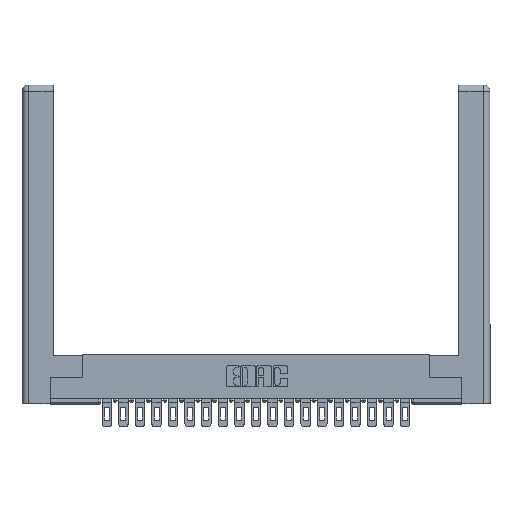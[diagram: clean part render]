
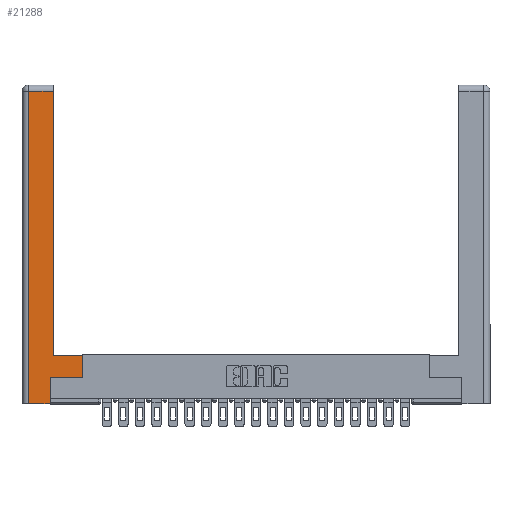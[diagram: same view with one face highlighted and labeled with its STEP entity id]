
A CAD part, top view. The second image highlights one B-rep face of the part: STEP entity #21288.
In plain terms, the highlighted planar face has unit normal (0, 0, 1).
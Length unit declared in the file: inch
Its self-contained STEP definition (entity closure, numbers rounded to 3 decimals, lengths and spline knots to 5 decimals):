
#2 = EDGE_CURVE ( 'NONE', #5353, #17691, #2559, .T. ) ;
#221 = ORIENTED_EDGE ( 'NONE', *, *, #21952, .T. ) ;
#541 = EDGE_CURVE ( 'NONE', #5933, #18225, #8132, .T. ) ;
#936 = VECTOR ( 'NONE', #11601, 39.37008 ) ;
#969 = CARTESIAN_POINT ( 'NONE',  ( 0.0615, 2.94, 0. ) ) ;
#1116 = LINE ( 'NONE', #15059, #15071 ) ;
#1229 = LINE ( 'NONE', #8319, #14444 ) ;
#1489 = CARTESIAN_POINT ( 'NONE',  ( 0.295, 2.94, 0. ) ) ;
#1703 = VECTOR ( 'NONE', #14948, 39.37008 ) ;
#2006 = ORIENTED_EDGE ( 'NONE', *, *, #16409, .T. ) ;
#2559 = LINE ( 'NONE', #12958, #22530 ) ;
#3538 = EDGE_CURVE ( 'NONE', #9638, #11837, #21744, .T. ) ;
#4379 = DIRECTION ( 'NONE',  ( 0., 1., 0. ) ) ;
#4420 = CARTESIAN_POINT ( 'NONE',  ( 0.565, 0.245, 0. ) ) ;
#4484 = CARTESIAN_POINT ( 'NONE',  ( 0.265, 0., 0. ) ) ;
#4649 = CARTESIAN_POINT ( 'NONE',  ( 0.265, 0.245, 0. ) ) ;
#5353 = VERTEX_POINT ( 'NONE', #4420 ) ;
#5506 = CARTESIAN_POINT ( 'NONE',  ( 0.565, 0.45, 0. ) ) ;
#5794 = ORIENTED_EDGE ( 'NONE', *, *, #19524, .T. ) ;
#5933 = VERTEX_POINT ( 'NONE', #22393 ) ;
#6152 = CARTESIAN_POINT ( 'NONE',  ( 0.265, 0., 0. ) ) ;
#7024 = DIRECTION ( 'NONE',  ( 0., 0., -1. ) ) ;
#8132 = LINE ( 'NONE', #4484, #17744 ) ;
#8298 = LINE ( 'NONE', #20510, #1703 ) ;
#8319 = CARTESIAN_POINT ( 'NONE',  ( 0.565, 0.245, 0. ) ) ;
#8575 = VECTOR ( 'NONE', #18726, 39.37008 ) ;
#8745 = PLANE ( 'NONE',  #9283 ) ;
#9079 = CARTESIAN_POINT ( 'NONE',  ( 0., 0., 0. ) ) ;
#9283 = AXIS2_PLACEMENT_3D ( 'NONE', #9079, #7024, #10326 ) ;
#9603 = CARTESIAN_POINT ( 'NONE',  ( 0.0615, 2.94, 0. ) ) ;
#9638 = VERTEX_POINT ( 'NONE', #1489 ) ;
#9863 = ORIENTED_EDGE ( 'NONE', *, *, #3538, .T. ) ;
#10326 = DIRECTION ( 'NONE',  ( -1., 0., 0. ) ) ;
#11444 = DIRECTION ( 'NONE',  ( 1., 0., 0. ) ) ;
#11601 = DIRECTION ( 'NONE',  ( 0., 1., 0. ) ) ;
#11837 = VERTEX_POINT ( 'NONE', #9603 ) ;
#12423 = ORIENTED_EDGE ( 'NONE', *, *, #22442, .T. ) ;
#12958 = CARTESIAN_POINT ( 'NONE',  ( 0.565, 0.45, 0. ) ) ;
#13187 = DIRECTION ( 'NONE',  ( -1., 0., 0. ) ) ;
#13494 = LINE ( 'NONE', #14892, #8575 ) ;
#14247 = LINE ( 'NONE', #21192, #936 ) ;
#14255 = ORIENTED_EDGE ( 'NONE', *, *, #15371, .T. ) ;
#14444 = VECTOR ( 'NONE', #18371, 39.37008 ) ;
#14892 = CARTESIAN_POINT ( 'NONE',  ( 0.295, 0.45, 0. ) ) ;
#14948 = DIRECTION ( 'NONE',  ( 0., -1., 0. ) ) ;
#15001 = VERTEX_POINT ( 'NONE', #21662 ) ;
#15034 = VERTEX_POINT ( 'NONE', #4649 ) ;
#15059 = CARTESIAN_POINT ( 'NONE',  ( 0.265, 0.245, 0. ) ) ;
#15071 = VECTOR ( 'NONE', #21999, 39.37008 ) ;
#15136 = VECTOR ( 'NONE', #13187, 39.37008 ) ;
#15371 = EDGE_CURVE ( 'NONE', #15001, #9638, #14247, .T. ) ;
#15726 = FACE_OUTER_BOUND ( 'NONE', #18541, .T. ) ;
#16409 = EDGE_CURVE ( 'NONE', #11837, #5933, #8298, .T. ) ;
#16523 = ORIENTED_EDGE ( 'NONE', *, *, #541, .T. ) ;
#17691 = VERTEX_POINT ( 'NONE', #5506 ) ;
#17744 = VECTOR ( 'NONE', #11444, 39.37008 ) ;
#18225 = VERTEX_POINT ( 'NONE', #6152 ) ;
#18371 = DIRECTION ( 'NONE',  ( 1., 0., 0. ) ) ;
#18541 = EDGE_LOOP ( 'NONE', ( #14255, #9863, #2006, #16523, #5794, #12423, #19025, #221 ) ) ;
#18726 = DIRECTION ( 'NONE',  ( -1., 0., 0. ) ) ;
#19025 = ORIENTED_EDGE ( 'NONE', *, *, #2, .T. ) ;
#19524 = EDGE_CURVE ( 'NONE', #18225, #15034, #1116, .T. ) ;
#20510 = CARTESIAN_POINT ( 'NONE',  ( 0.0615, 0., 0. ) ) ;
#21192 = CARTESIAN_POINT ( 'NONE',  ( 0.295, 3., 0. ) ) ;
#21288 = ADVANCED_FACE ( 'NONE', ( #15726 ), #8745, .F. ) ;
#21662 = CARTESIAN_POINT ( 'NONE',  ( 0.295, 0.45, 0. ) ) ;
#21744 = LINE ( 'NONE', #969, #15136 ) ;
#21952 = EDGE_CURVE ( 'NONE', #17691, #15001, #13494, .T. ) ;
#21999 = DIRECTION ( 'NONE',  ( 0., 1., 0. ) ) ;
#22393 = CARTESIAN_POINT ( 'NONE',  ( 0.0615, 0., 0. ) ) ;
#22442 = EDGE_CURVE ( 'NONE', #15034, #5353, #1229, .T. ) ;
#22530 = VECTOR ( 'NONE', #4379, 39.37008 ) ;
